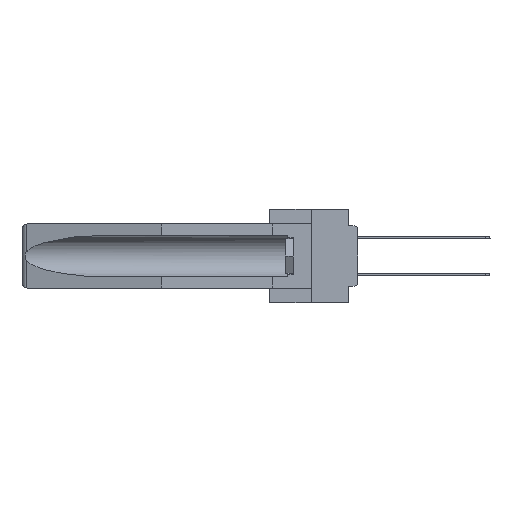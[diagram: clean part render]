
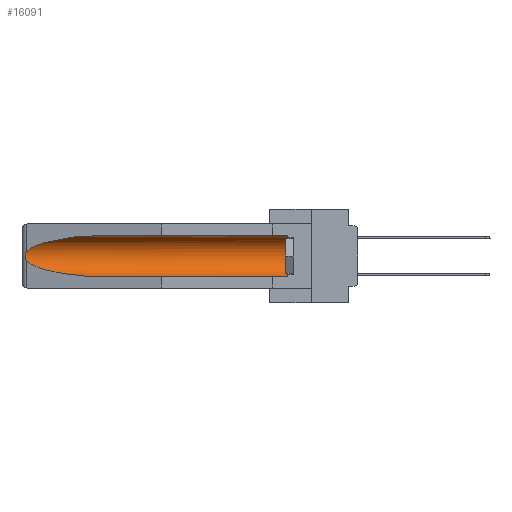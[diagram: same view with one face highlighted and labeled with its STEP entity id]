
A CAD part, left-side view. The second image highlights one B-rep face of the part: STEP entity #16091.
In plain terms, the highlighted cylindrical face has radius 2.857 mm (diameter 5.715 mm), a partial arc.
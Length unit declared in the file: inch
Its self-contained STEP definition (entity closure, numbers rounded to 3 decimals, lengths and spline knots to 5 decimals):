
#68 = CARTESIAN_POINT ( 'NONE',  ( 0.155, 1.07973, -0.284 ) ) ;
#2306 = CARTESIAN_POINT ( 'NONE',  ( 0.155, 0.126, -0.284 ) ) ;
#3162 = CARTESIAN_POINT ( 'NONE',  ( 0.26597, 1.52961, -0.15275 ) ) ;
#5381 = CARTESIAN_POINT ( 'NONE',  ( 0.155, 1.07973, -0.059 ) ) ;
#5809 = ORIENTED_EDGE ( 'NONE', *, *, #7879, .T. ) ;
#5814 = CARTESIAN_POINT ( 'NONE',  ( 0.155, 0.126, -0.1715 ) ) ;
#5816 = CARTESIAN_POINT ( 'NONE',  ( 0.26654, 1.53092, -0.15636 ) ) ;
#7157 = EDGE_CURVE ( 'NONE', #18850, #30688, #9150, .T. ) ;
#7199 = CARTESIAN_POINT ( 'NONE',  ( 0.26537, 1.52718, -0.19328 ) ) ;
#7879 = EDGE_CURVE ( 'NONE', #28248, #30688, #21567, .T. ) ;
#8616 = CARTESIAN_POINT ( 'NONE',  ( 0.2673, 1.5327, -0.16383 ) ) ;
#9150 = LINE ( 'NONE', #25610, #15901 ) ;
#10061 = AXIS2_PLACEMENT_3D ( 'NONE', #5814, #28937, #34641 ) ;
#10133 = ORIENTED_EDGE ( 'NONE', *, *, #17735, .T. ) ;
#10263 = CARTESIAN_POINT ( 'NONE',  ( 0.155, 1.07973, -0.284 ) ) ;
#10339 = VERTEX_POINT ( 'NONE', #5381 ) ;
#11129 = AXIS2_PLACEMENT_3D ( 'NONE', #36055, #24254, #21578 ) ;
#11488 =( BOUNDED_CURVE ( )  B_SPLINE_CURVE ( 3, ( #34342, #14020, #37155, #19791 ),
 .UNSPECIFIED., .F., .F. ) 
 B_SPLINE_CURVE_WITH_KNOTS ( ( 4, 4 ),
 ( 4.71239, 6.08839 ),
 .UNSPECIFIED. ) 
 CURVE ( )  GEOMETRIC_REPRESENTATION_ITEM ( )  RATIONAL_B_SPLINE_CURVE ( ( 1., 0.848, 0.848, 1. ) ) 
 REPRESENTATION_ITEM ( '' )  );
#11935 = CARTESIAN_POINT ( 'NONE',  ( 0.2675, 1.53308, -0.17534 ) ) ;
#12892 = ORIENTED_EDGE ( 'NONE', *, *, #20892, .T. ) ;
#14020 = CARTESIAN_POINT ( 'NONE',  ( 0.21114, 1.30732, -0.059 ) ) ;
#14245 = VERTEX_POINT ( 'NONE', #29521 ) ;
#14558 = CARTESIAN_POINT ( 'NONE',  ( 0.26597, 1.5296, -0.19026 ) ) ;
#15420 = CARTESIAN_POINT ( 'NONE',  ( 0.21114, 1.30732, -0.284 ) ) ;
#15815 = B_SPLINE_CURVE_WITH_KNOTS ( 'NONE', 3,
 ( #23088, #3162, #5816, #8616, #23211, #11935, #17655, #25755, #14558, #28803 ),
 .UNSPECIFIED., .F., .F.,
 ( 4, 2, 2, 2, 4 ),
 ( 0., 0.00029, 0.00058, 0.00087, 0.00117 ),
 .UNSPECIFIED. ) ;
#15901 = VECTOR ( 'NONE', #28524, 39.37008 ) ;
#16091 = ADVANCED_FACE ( 'NONE', ( #18793 ), #33274, .F. ) ;
#17655 = CARTESIAN_POINT ( 'NONE',  ( 0.2673, 1.53269, -0.17917 ) ) ;
#17735 = EDGE_CURVE ( 'NONE', #10339, #31313, #11488, .T. ) ;
#17824 = ORIENTED_EDGE ( 'NONE', *, *, #25498, .T. ) ;
#18793 = FACE_OUTER_BOUND ( 'NONE', #22541, .T. ) ;
#18850 = VERTEX_POINT ( 'NONE', #2306 ) ;
#19791 = CARTESIAN_POINT ( 'NONE',  ( 0.26537, 1.52718, -0.14972 ) ) ;
#20874 = CIRCLE ( 'NONE', #10061, 0.1125 ) ;
#20892 = EDGE_CURVE ( 'NONE', #31313, #28248, #15815, .T. ) ;
#21567 =( BOUNDED_CURVE ( )  B_SPLINE_CURVE ( 3, ( #7199, #32732, #15420, #10263 ),
 .UNSPECIFIED., .F., .F. ) 
 B_SPLINE_CURVE_WITH_KNOTS ( ( 4, 4 ),
 ( 0.1948, 1.5708 ),
 .UNSPECIFIED. ) 
 CURVE ( )  GEOMETRIC_REPRESENTATION_ITEM ( )  RATIONAL_B_SPLINE_CURVE ( ( 1., 0.848, 0.848, 1. ) ) 
 REPRESENTATION_ITEM ( '' )  );
#21578 = DIRECTION ( 'NONE',  ( 0., 0., 1. ) ) ;
#22541 = EDGE_LOOP ( 'NONE', ( #10133, #12892, #5809, #31642, #17824, #29060 ) ) ;
#23088 = CARTESIAN_POINT ( 'NONE',  ( 0.26537, 1.52718, -0.14972 ) ) ;
#23211 = CARTESIAN_POINT ( 'NONE',  ( 0.2675, 1.53308, -0.16763 ) ) ;
#24254 = DIRECTION ( 'NONE',  ( 0., 1., 0. ) ) ;
#25498 = EDGE_CURVE ( 'NONE', #18850, #14245, #20874, .T. ) ;
#25610 = CARTESIAN_POINT ( 'NONE',  ( 0.155, -0.30754, -0.284 ) ) ;
#25755 = CARTESIAN_POINT ( 'NONE',  ( 0.26655, 1.53094, -0.18657 ) ) ;
#26021 = LINE ( 'NONE', #27071, #31912 ) ;
#27071 = CARTESIAN_POINT ( 'NONE',  ( 0.155, -0.30754, -0.059 ) ) ;
#27330 = DIRECTION ( 'NONE',  ( 0., 1., 0. ) ) ;
#28248 = VERTEX_POINT ( 'NONE', #36506 ) ;
#28524 = DIRECTION ( 'NONE',  ( 0., 1., 0. ) ) ;
#28803 = CARTESIAN_POINT ( 'NONE',  ( 0.26537, 1.52718, -0.19328 ) ) ;
#28937 = DIRECTION ( 'NONE',  ( 0., -1., 0. ) ) ;
#29060 = ORIENTED_EDGE ( 'NONE', *, *, #30967, .T. ) ;
#29521 = CARTESIAN_POINT ( 'NONE',  ( 0.155, 0.126, -0.059 ) ) ;
#30688 = VERTEX_POINT ( 'NONE', #68 ) ;
#30967 = EDGE_CURVE ( 'NONE', #14245, #10339, #26021, .T. ) ;
#31313 = VERTEX_POINT ( 'NONE', #34050 ) ;
#31642 = ORIENTED_EDGE ( 'NONE', *, *, #7157, .F. ) ;
#31912 = VECTOR ( 'NONE', #27330, 39.37008 ) ;
#32732 = CARTESIAN_POINT ( 'NONE',  ( 0.25451, 1.48313, -0.24835 ) ) ;
#33274 = CYLINDRICAL_SURFACE ( 'NONE', #11129, 0.1125 ) ;
#34050 = CARTESIAN_POINT ( 'NONE',  ( 0.26537, 1.52718, -0.14972 ) ) ;
#34342 = CARTESIAN_POINT ( 'NONE',  ( 0.155, 1.07973, -0.059 ) ) ;
#34641 = DIRECTION ( 'NONE',  ( 0., 0., 1. ) ) ;
#36055 = CARTESIAN_POINT ( 'NONE',  ( 0.155, -0.30754, -0.1715 ) ) ;
#36506 = CARTESIAN_POINT ( 'NONE',  ( 0.26537, 1.52718, -0.19328 ) ) ;
#37155 = CARTESIAN_POINT ( 'NONE',  ( 0.25451, 1.48313, -0.09465 ) ) ;
